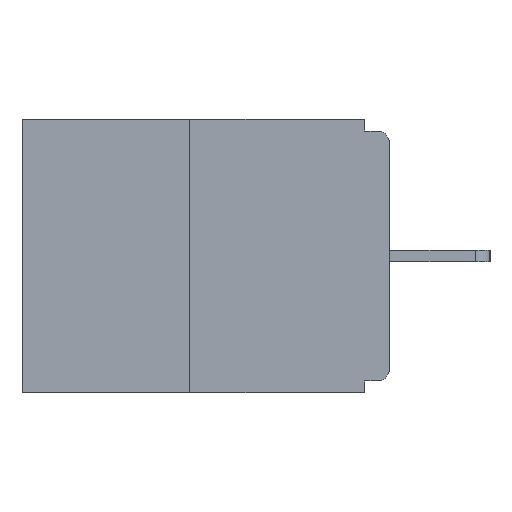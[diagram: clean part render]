
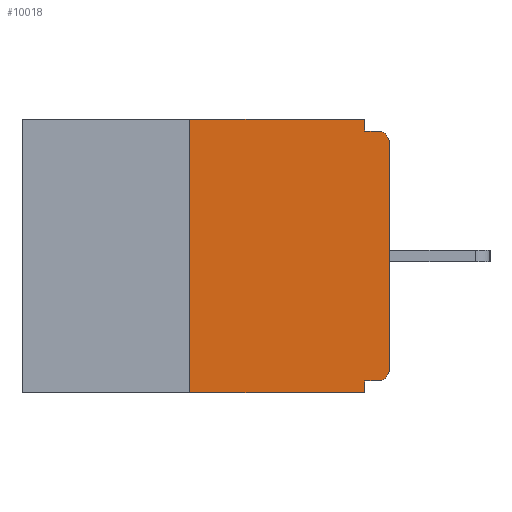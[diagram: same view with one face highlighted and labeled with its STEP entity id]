
A CAD part, left-side view. The second image highlights one B-rep face of the part: STEP entity #10018.
In plain terms, the highlighted planar face has unit normal (-1, 0, 0).
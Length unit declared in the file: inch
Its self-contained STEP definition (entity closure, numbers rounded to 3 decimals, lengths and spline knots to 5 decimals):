
#608 = DIRECTION ( 'NONE',  ( -1., 0., 0. ) ) ;
#639 = VECTOR ( 'NONE', #6203, 39.37008 ) ;
#828 = LINE ( 'NONE', #12939, #7211 ) ;
#936 = LINE ( 'NONE', #12134, #7667 ) ;
#1055 = VERTEX_POINT ( 'NONE', #4707 ) ;
#1525 = VECTOR ( 'NONE', #9602, 39.37008 ) ;
#2107 = DIRECTION ( 'NONE',  ( 0., -1., 0. ) ) ;
#2595 = DIRECTION ( 'NONE',  ( -1., 0., 0. ) ) ;
#2804 = ORIENTED_EDGE ( 'NONE', *, *, #6718, .F. ) ;
#2903 = ORIENTED_EDGE ( 'NONE', *, *, #6659, .T. ) ;
#3023 = DIRECTION ( 'NONE',  ( 0., 0., -1. ) ) ;
#3036 = CARTESIAN_POINT ( 'NONE',  ( 0., 0.46, -0.343 ) ) ;
#3062 = ORIENTED_EDGE ( 'NONE', *, *, #6759, .F. ) ;
#3104 = VECTOR ( 'NONE', #7741, 39.37008 ) ;
#3151 = PLANE ( 'NONE',  #5692 ) ;
#3503 = CARTESIAN_POINT ( 'NONE',  ( 0., 0.25, 0. ) ) ;
#3891 = CARTESIAN_POINT ( 'NONE',  ( 0., 0., -0.313 ) ) ;
#3920 = DIRECTION ( 'NONE',  ( 0., -1., 0. ) ) ;
#4100 = ORIENTED_EDGE ( 'NONE', *, *, #7223, .F. ) ;
#4130 = FACE_OUTER_BOUND ( 'NONE', #6216, .T. ) ;
#4707 = CARTESIAN_POINT ( 'NONE',  ( 0., 0.031, -0.328 ) ) ;
#4819 = LINE ( 'NONE', #12899, #3104 ) ;
#4955 = CARTESIAN_POINT ( 'NONE',  ( 0., 0.031, -0.343 ) ) ;
#4991 = CARTESIAN_POINT ( 'NONE',  ( 0., 0.25, 0. ) ) ;
#5018 = LINE ( 'NONE', #4955, #8929 ) ;
#5159 = LINE ( 'NONE', #3036, #11995 ) ;
#5257 = CARTESIAN_POINT ( 'NONE',  ( 0., 0., -0.328 ) ) ;
#5567 = ORIENTED_EDGE ( 'NONE', *, *, #12110, .F. ) ;
#5633 = CARTESIAN_POINT ( 'NONE',  ( 0., 0.015, -0.015 ) ) ;
#5692 = AXIS2_PLACEMENT_3D ( 'NONE', #9982, #11256, #3023 ) ;
#5768 = EDGE_CURVE ( 'NONE', #9525, #8948, #11456, .T. ) ;
#5889 = VERTEX_POINT ( 'NONE', #12874 ) ;
#6005 = VERTEX_POINT ( 'NONE', #7144 ) ;
#6186 = ORIENTED_EDGE ( 'NONE', *, *, #8289, .T. ) ;
#6203 = DIRECTION ( 'NONE',  ( 0., 1., 0. ) ) ;
#6216 = EDGE_LOOP ( 'NONE', ( #11455, #2804, #6186, #4100, #9879, #10080, #7849, #2903, #5567, #3062 ) ) ;
#6659 = EDGE_CURVE ( 'NONE', #8948, #10613, #9556, .T. ) ;
#6718 = EDGE_CURVE ( 'NONE', #7291, #12292, #12589, .T. ) ;
#6759 = EDGE_CURVE ( 'NONE', #10212, #12655, #936, .T. ) ;
#6846 = CARTESIAN_POINT ( 'NONE',  ( 0., 0.25, -0.343 ) ) ;
#7144 = CARTESIAN_POINT ( 'NONE',  ( 0., 0.031, -0.343 ) ) ;
#7211 = VECTOR ( 'NONE', #3920, 39.37008 ) ;
#7223 = EDGE_CURVE ( 'NONE', #1055, #6005, #5018, .T. ) ;
#7291 = VERTEX_POINT ( 'NONE', #6846 ) ;
#7292 = DIRECTION ( 'NONE',  ( 0., 0., 1. ) ) ;
#7667 = VECTOR ( 'NONE', #10866, 39.37008 ) ;
#7741 = DIRECTION ( 'NONE',  ( 0., -1., 0. ) ) ;
#7849 = ORIENTED_EDGE ( 'NONE', *, *, #5768, .T. ) ;
#7887 = DIRECTION ( 'NONE',  ( 0., 0., -1. ) ) ;
#8151 = EDGE_CURVE ( 'NONE', #12292, #10212, #4819, .T. ) ;
#8208 = AXIS2_PLACEMENT_3D ( 'NONE', #12791, #2595, #8756 ) ;
#8289 = EDGE_CURVE ( 'NONE', #7291, #6005, #5159, .T. ) ;
#8486 = VECTOR ( 'NONE', #7292, 39.37008 ) ;
#8620 = CIRCLE ( 'NONE', #8208, 0.015 ) ;
#8756 = DIRECTION ( 'NONE',  ( 0., 0., -1. ) ) ;
#8929 = VECTOR ( 'NONE', #7887, 39.37008 ) ;
#8948 = VERTEX_POINT ( 'NONE', #11311 ) ;
#9132 = CARTESIAN_POINT ( 'NONE',  ( 0., 0.031, -0.015 ) ) ;
#9342 = AXIS2_PLACEMENT_3D ( 'NONE', #10661, #608, #11601 ) ;
#9525 = VERTEX_POINT ( 'NONE', #3891 ) ;
#9556 = CIRCLE ( 'NONE', #9342, 0.015 ) ;
#9602 = DIRECTION ( 'NONE',  ( 0., 0., 1. ) ) ;
#9618 = CARTESIAN_POINT ( 'NONE',  ( 0., 0.031, 0. ) ) ;
#9879 = ORIENTED_EDGE ( 'NONE', *, *, #12256, .F. ) ;
#9982 = CARTESIAN_POINT ( 'NONE',  ( 0., 0.46, 0. ) ) ;
#10018 = ADVANCED_FACE ( 'NONE', ( #4130 ), #3151, .F. ) ;
#10080 = ORIENTED_EDGE ( 'NONE', *, *, #10205, .T. ) ;
#10205 = EDGE_CURVE ( 'NONE', #5889, #9525, #8620, .T. ) ;
#10212 = VERTEX_POINT ( 'NONE', #9618 ) ;
#10435 = CARTESIAN_POINT ( 'NONE',  ( 0., 0., 0. ) ) ;
#10613 = VERTEX_POINT ( 'NONE', #5633 ) ;
#10661 = CARTESIAN_POINT ( 'NONE',  ( 0., 0.015, -0.03 ) ) ;
#10866 = DIRECTION ( 'NONE',  ( 0., 0., -1. ) ) ;
#11256 = DIRECTION ( 'NONE',  ( 1., 0., 0. ) ) ;
#11311 = CARTESIAN_POINT ( 'NONE',  ( 0., 0., -0.03 ) ) ;
#11455 = ORIENTED_EDGE ( 'NONE', *, *, #8151, .F. ) ;
#11456 = LINE ( 'NONE', #10435, #8486 ) ;
#11601 = DIRECTION ( 'NONE',  ( 0., 0., -1. ) ) ;
#11995 = VECTOR ( 'NONE', #2107, 39.37008 ) ;
#12110 = EDGE_CURVE ( 'NONE', #12655, #10613, #828, .T. ) ;
#12134 = CARTESIAN_POINT ( 'NONE',  ( 0., 0.031, 0. ) ) ;
#12158 = LINE ( 'NONE', #5257, #639 ) ;
#12256 = EDGE_CURVE ( 'NONE', #5889, #1055, #12158, .T. ) ;
#12292 = VERTEX_POINT ( 'NONE', #4991 ) ;
#12589 = LINE ( 'NONE', #3503, #1525 ) ;
#12655 = VERTEX_POINT ( 'NONE', #9132 ) ;
#12791 = CARTESIAN_POINT ( 'NONE',  ( 0., 0.015, -0.313 ) ) ;
#12874 = CARTESIAN_POINT ( 'NONE',  ( 0., 0.015, -0.328 ) ) ;
#12899 = CARTESIAN_POINT ( 'NONE',  ( 0., 0.46, 0. ) ) ;
#12939 = CARTESIAN_POINT ( 'NONE',  ( 0., 0., -0.015 ) ) ;
